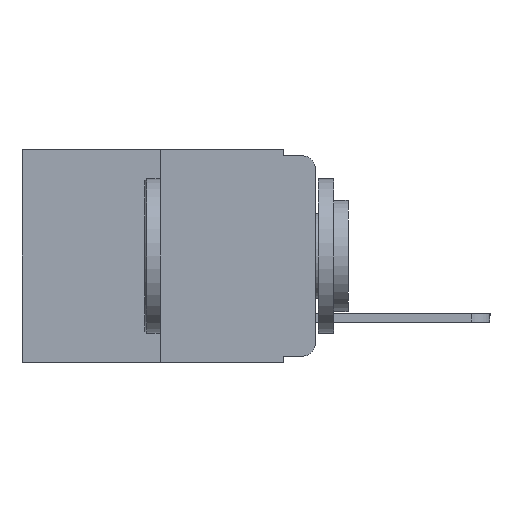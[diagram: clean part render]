
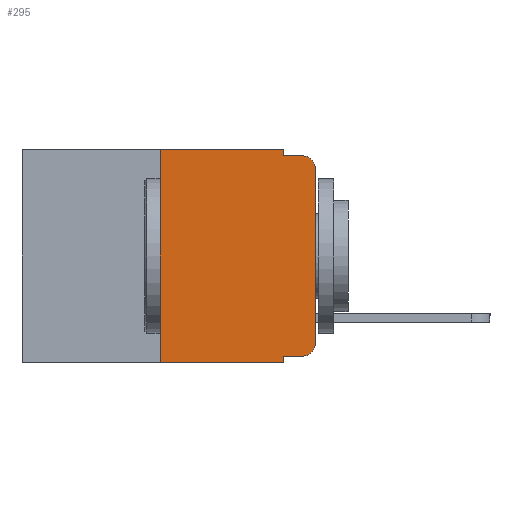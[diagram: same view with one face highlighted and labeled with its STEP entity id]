
A CAD part, left-side view. The second image highlights one B-rep face of the part: STEP entity #295.
In plain terms, the highlighted planar face has unit normal (-1, 0, 0).
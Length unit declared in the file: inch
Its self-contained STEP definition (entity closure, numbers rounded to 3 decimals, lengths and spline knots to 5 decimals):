
#53 = VECTOR ( 'NONE', #13022, 39.37008 ) ;
#87 = EDGE_LOOP ( 'NONE', ( #6891, #8376, #9838, #5466, #3493, #11076, #653, #1751, #5120, #9298 ) ) ;
#295 = ADVANCED_FACE ( 'NONE', ( #661 ), #8110, .F. ) ;
#409 = EDGE_CURVE ( 'NONE', #11955, #3670, #8399, .T. ) ;
#466 = CARTESIAN_POINT ( 'NONE',  ( 0., 0.473, 0. ) ) ;
#653 = ORIENTED_EDGE ( 'NONE', *, *, #9511, .T. ) ;
#661 = FACE_OUTER_BOUND ( 'NONE', #87, .T. ) ;
#754 = LINE ( 'NONE', #7876, #3421 ) ;
#987 = DIRECTION ( 'NONE',  ( 0., -1., 0. ) ) ;
#1349 = CARTESIAN_POINT ( 'NONE',  ( 0., 0.051, -0.01 ) ) ;
#1751 = ORIENTED_EDGE ( 'NONE', *, *, #10224, .F. ) ;
#2558 = LINE ( 'NONE', #3256, #11719 ) ;
#2655 = DIRECTION ( 'NONE',  ( 0., 0., 1. ) ) ;
#2785 = DIRECTION ( 'NONE',  ( 0., -1., 0. ) ) ;
#3092 = DIRECTION ( 'NONE',  ( 1., 0., 0. ) ) ;
#3256 = CARTESIAN_POINT ( 'NONE',  ( 0., 0.051, -0.333 ) ) ;
#3295 = CARTESIAN_POINT ( 'NONE',  ( 0., 0.051, -0.343 ) ) ;
#3421 = VECTOR ( 'NONE', #987, 39.37008 ) ;
#3493 = ORIENTED_EDGE ( 'NONE', *, *, #9535, .F. ) ;
#3615 = DIRECTION ( 'NONE',  ( 0., 0., -1. ) ) ;
#3656 = CARTESIAN_POINT ( 'NONE',  ( 0., 0.02, -0.03 ) ) ;
#3670 = VERTEX_POINT ( 'NONE', #1349 ) ;
#3901 = DIRECTION ( 'NONE',  ( 0., 0., 1. ) ) ;
#4818 = DIRECTION ( 'NONE',  ( 0., 0., -1. ) ) ;
#4958 = CARTESIAN_POINT ( 'NONE',  ( 0., 0.02, -0.01 ) ) ;
#5067 = AXIS2_PLACEMENT_3D ( 'NONE', #13254, #6418, #14397 ) ;
#5120 = ORIENTED_EDGE ( 'NONE', *, *, #10683, .T. ) ;
#5432 = AXIS2_PLACEMENT_3D ( 'NONE', #14767, #3092, #13443 ) ;
#5466 = ORIENTED_EDGE ( 'NONE', *, *, #409, .F. ) ;
#5610 = VERTEX_POINT ( 'NONE', #4958 ) ;
#5635 = CARTESIAN_POINT ( 'NONE',  ( 0., 0., -0.03 ) ) ;
#5911 = LINE ( 'NONE', #8394, #12028 ) ;
#6125 = LINE ( 'NONE', #13505, #14529 ) ;
#6418 = DIRECTION ( 'NONE',  ( -1., 0., 0. ) ) ;
#6891 = ORIENTED_EDGE ( 'NONE', *, *, #12241, .T. ) ;
#7755 = VERTEX_POINT ( 'NONE', #14171 ) ;
#7829 = CARTESIAN_POINT ( 'NONE',  ( 0., 0.051, 0. ) ) ;
#7876 = CARTESIAN_POINT ( 'NONE',  ( 0., 0.051, -0.01 ) ) ;
#7904 = DIRECTION ( 'NONE',  ( 0., 0., -1. ) ) ;
#8083 = LINE ( 'NONE', #9681, #11143 ) ;
#8110 = PLANE ( 'NONE',  #5432 ) ;
#8376 = ORIENTED_EDGE ( 'NONE', *, *, #9804, .T. ) ;
#8394 = CARTESIAN_POINT ( 'NONE',  ( 0., 0.25, 0. ) ) ;
#8399 = LINE ( 'NONE', #7829, #13712 ) ;
#8553 = CARTESIAN_POINT ( 'NONE',  ( 0., 0.02, -0.333 ) ) ;
#9170 = CARTESIAN_POINT ( 'NONE',  ( 0., 0.051, 0. ) ) ;
#9240 = LINE ( 'NONE', #466, #14547 ) ;
#9298 = ORIENTED_EDGE ( 'NONE', *, *, #13329, .T. ) ;
#9511 = EDGE_CURVE ( 'NONE', #11059, #10721, #12249, .T. ) ;
#9535 = EDGE_CURVE ( 'NONE', #7755, #11955, #9240, .T. ) ;
#9681 = CARTESIAN_POINT ( 'NONE',  ( 0., 0., 0. ) ) ;
#9711 = AXIS2_PLACEMENT_3D ( 'NONE', #3656, #11714, #4818 ) ;
#9804 = EDGE_CURVE ( 'NONE', #13563, #5610, #11363, .T. ) ;
#9838 = ORIENTED_EDGE ( 'NONE', *, *, #11278, .F. ) ;
#10224 = EDGE_CURVE ( 'NONE', #11589, #10721, #6125, .T. ) ;
#10683 = EDGE_CURVE ( 'NONE', #11589, #13884, #2558, .T. ) ;
#10721 = VERTEX_POINT ( 'NONE', #3295 ) ;
#10734 = CARTESIAN_POINT ( 'NONE',  ( 0., 0., -0.313 ) ) ;
#10794 = CARTESIAN_POINT ( 'NONE',  ( 0., 0.051, -0.333 ) ) ;
#11059 = VERTEX_POINT ( 'NONE', #12020 ) ;
#11076 = ORIENTED_EDGE ( 'NONE', *, *, #13797, .F. ) ;
#11143 = VECTOR ( 'NONE', #3901, 39.37008 ) ;
#11278 = EDGE_CURVE ( 'NONE', #3670, #5610, #754, .T. ) ;
#11363 = CIRCLE ( 'NONE', #9711, 0.02 ) ;
#11589 = VERTEX_POINT ( 'NONE', #10794 ) ;
#11714 = DIRECTION ( 'NONE',  ( -1., 0., 0. ) ) ;
#11719 = VECTOR ( 'NONE', #14676, 39.37008 ) ;
#11893 = CARTESIAN_POINT ( 'NONE',  ( 0., 0.473, -0.343 ) ) ;
#11955 = VERTEX_POINT ( 'NONE', #9170 ) ;
#12020 = CARTESIAN_POINT ( 'NONE',  ( 0., 0.25, -0.343 ) ) ;
#12028 = VECTOR ( 'NONE', #2655, 39.37008 ) ;
#12042 = CIRCLE ( 'NONE', #5067, 0.02 ) ;
#12241 = EDGE_CURVE ( 'NONE', #14450, #13563, #8083, .T. ) ;
#12249 = LINE ( 'NONE', #11893, #53 ) ;
#13022 = DIRECTION ( 'NONE',  ( 0., -1., 0. ) ) ;
#13254 = CARTESIAN_POINT ( 'NONE',  ( 0., 0.02, -0.313 ) ) ;
#13329 = EDGE_CURVE ( 'NONE', #13884, #14450, #12042, .T. ) ;
#13443 = DIRECTION ( 'NONE',  ( 0., 0., -1. ) ) ;
#13505 = CARTESIAN_POINT ( 'NONE',  ( 0., 0.051, 0. ) ) ;
#13563 = VERTEX_POINT ( 'NONE', #5635 ) ;
#13712 = VECTOR ( 'NONE', #3615, 39.37008 ) ;
#13797 = EDGE_CURVE ( 'NONE', #11059, #7755, #5911, .T. ) ;
#13884 = VERTEX_POINT ( 'NONE', #8553 ) ;
#14171 = CARTESIAN_POINT ( 'NONE',  ( 0., 0.25, 0. ) ) ;
#14397 = DIRECTION ( 'NONE',  ( 0., 0., -1. ) ) ;
#14450 = VERTEX_POINT ( 'NONE', #10734 ) ;
#14529 = VECTOR ( 'NONE', #7904, 39.37008 ) ;
#14547 = VECTOR ( 'NONE', #2785, 39.37008 ) ;
#14676 = DIRECTION ( 'NONE',  ( 0., -1., 0. ) ) ;
#14767 = CARTESIAN_POINT ( 'NONE',  ( 0., 0.473, 0. ) ) ;
